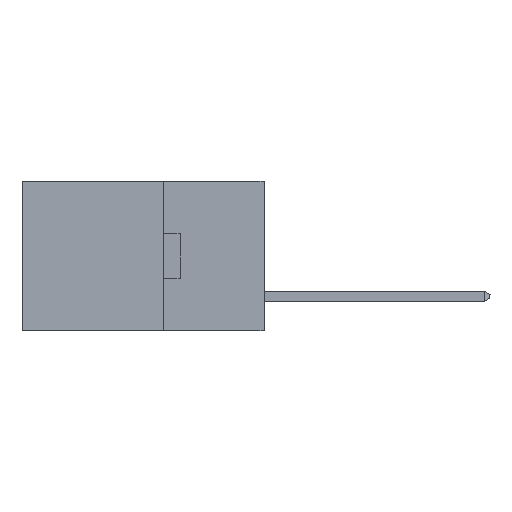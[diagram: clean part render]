
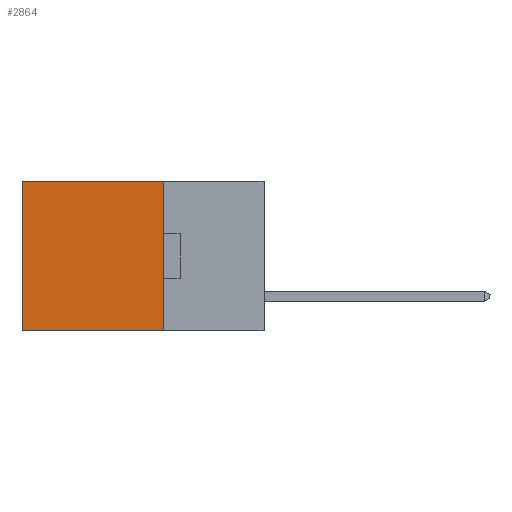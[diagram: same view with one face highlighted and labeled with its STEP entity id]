
A CAD part, left-side view. The second image highlights one B-rep face of the part: STEP entity #2864.
In plain terms, the highlighted planar face has unit normal (-1, 0, 0).
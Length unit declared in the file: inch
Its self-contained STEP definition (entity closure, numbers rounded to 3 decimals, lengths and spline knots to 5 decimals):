
#446 = LINE ( 'NONE', #25621, #14293 ) ;
#492 = VERTEX_POINT ( 'NONE', #26698 ) ;
#720 = CARTESIAN_POINT ( 'NONE',  ( 0.2615, 0.25, 0. ) ) ;
#2207 = LINE ( 'NONE', #6272, #24318 ) ;
#2235 = ORIENTED_EDGE ( 'NONE', *, *, #15915, .T. ) ;
#2468 = CARTESIAN_POINT ( 'NONE',  ( 0.2615, 0.6, 0. ) ) ;
#2864 = ADVANCED_FACE ( 'NONE', ( #25182 ), #14799, .F. ) ;
#4641 = LINE ( 'NONE', #720, #12255 ) ;
#5048 = VERTEX_POINT ( 'NONE', #12962 ) ;
#6112 = EDGE_CURVE ( 'NONE', #492, #13268, #11602, .T. ) ;
#6272 = CARTESIAN_POINT ( 'NONE',  ( 0.2615, 0.25, -0.37 ) ) ;
#6986 = VERTEX_POINT ( 'NONE', #2468 ) ;
#9579 = CARTESIAN_POINT ( 'NONE',  ( 0.2615, 0.25, -0.37 ) ) ;
#9606 = ORIENTED_EDGE ( 'NONE', *, *, #21503, .F. ) ;
#11160 = DIRECTION ( 'NONE',  ( 0., 0., -1. ) ) ;
#11602 = LINE ( 'NONE', #9579, #19612 ) ;
#12255 = VECTOR ( 'NONE', #19466, 39.37008 ) ;
#12962 = CARTESIAN_POINT ( 'NONE',  ( 0.2615, 0.6, -0.37 ) ) ;
#13018 = DIRECTION ( 'NONE',  ( 0., 0., -1. ) ) ;
#13268 = VERTEX_POINT ( 'NONE', #15556 ) ;
#14293 = VECTOR ( 'NONE', #11160, 39.37008 ) ;
#14799 = PLANE ( 'NONE',  #22610 ) ;
#15556 = CARTESIAN_POINT ( 'NONE',  ( 0.2615, 0.25, -0.37 ) ) ;
#15872 = EDGE_LOOP ( 'NONE', ( #20651, #9606, #22568, #2235 ) ) ;
#15915 = EDGE_CURVE ( 'NONE', #492, #6986, #4641, .T. ) ;
#17751 = DIRECTION ( 'NONE',  ( 0., 0., -1. ) ) ;
#19466 = DIRECTION ( 'NONE',  ( 0., 1., 0. ) ) ;
#19582 = DIRECTION ( 'NONE',  ( 1., 0., 0. ) ) ;
#19612 = VECTOR ( 'NONE', #17751, 39.37008 ) ;
#20651 = ORIENTED_EDGE ( 'NONE', *, *, #21684, .T. ) ;
#21503 = EDGE_CURVE ( 'NONE', #13268, #5048, #2207, .T. ) ;
#21684 = EDGE_CURVE ( 'NONE', #6986, #5048, #446, .T. ) ;
#22236 = DIRECTION ( 'NONE',  ( 0., 1., 0. ) ) ;
#22568 = ORIENTED_EDGE ( 'NONE', *, *, #6112, .F. ) ;
#22610 = AXIS2_PLACEMENT_3D ( 'NONE', #23130, #19582, #13018 ) ;
#23130 = CARTESIAN_POINT ( 'NONE',  ( 0.2615, 0.25, -0.37 ) ) ;
#24318 = VECTOR ( 'NONE', #22236, 39.37008 ) ;
#25182 = FACE_OUTER_BOUND ( 'NONE', #15872, .T. ) ;
#25621 = CARTESIAN_POINT ( 'NONE',  ( 0.2615, 0.6, -0.37 ) ) ;
#26698 = CARTESIAN_POINT ( 'NONE',  ( 0.2615, 0.25, 0. ) ) ;
